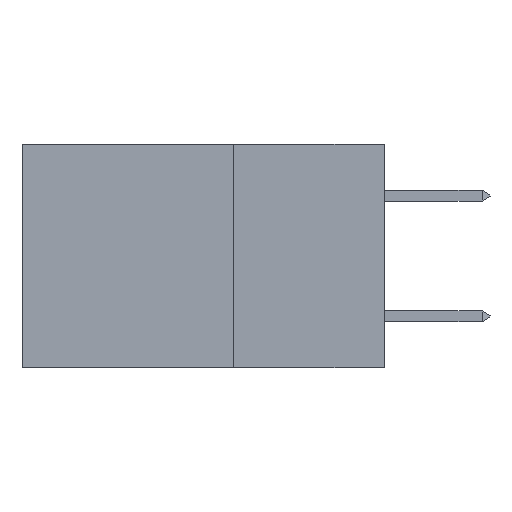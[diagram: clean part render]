
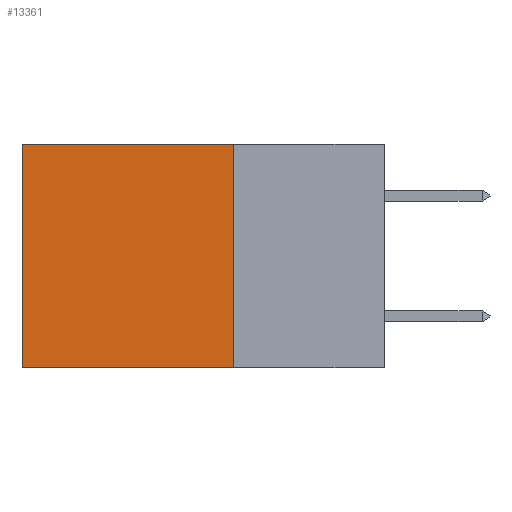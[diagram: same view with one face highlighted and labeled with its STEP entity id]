
A CAD part, left-side view. The second image highlights one B-rep face of the part: STEP entity #13361.
In plain terms, the highlighted planar face has unit normal (-1, 0, 0).
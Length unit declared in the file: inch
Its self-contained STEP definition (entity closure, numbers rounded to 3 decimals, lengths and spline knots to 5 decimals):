
#562 = PLANE ( 'NONE',  #2288 ) ;
#774 = DIRECTION ( 'NONE',  ( 0., 1., 0. ) ) ;
#834 = FACE_OUTER_BOUND ( 'NONE', #16332, .T. ) ;
#994 = ORIENTED_EDGE ( 'NONE', *, *, #23480, .T. ) ;
#1142 = VECTOR ( 'NONE', #774, 39.37008 ) ;
#2156 = CARTESIAN_POINT ( 'NONE',  ( 0.2875, 0.25, -0.37 ) ) ;
#2288 = AXIS2_PLACEMENT_3D ( 'NONE', #22268, #9350, #15527 ) ;
#2604 = CARTESIAN_POINT ( 'NONE',  ( 0.2875, 0.6, -0.37 ) ) ;
#4967 = CARTESIAN_POINT ( 'NONE',  ( 0.2875, 0.25, 0. ) ) ;
#6577 = CARTESIAN_POINT ( 'NONE',  ( 0.2875, 0.6, 0. ) ) ;
#6912 = VERTEX_POINT ( 'NONE', #2604 ) ;
#6978 = EDGE_CURVE ( 'NONE', #10164, #23298, #17303, .T. ) ;
#7109 = VECTOR ( 'NONE', #21839, 39.37008 ) ;
#7197 = VERTEX_POINT ( 'NONE', #2156 ) ;
#9350 = DIRECTION ( 'NONE',  ( 1., 0., 0. ) ) ;
#10164 = VERTEX_POINT ( 'NONE', #12067 ) ;
#11498 = ORIENTED_EDGE ( 'NONE', *, *, #21972, .F. ) ;
#12067 = CARTESIAN_POINT ( 'NONE',  ( 0.2875, 0.25, 0. ) ) ;
#12426 = VECTOR ( 'NONE', #22539, 39.37008 ) ;
#13188 = ORIENTED_EDGE ( 'NONE', *, *, #6978, .T. ) ;
#13361 = ADVANCED_FACE ( 'NONE', ( #834 ), #562, .F. ) ;
#13532 = CARTESIAN_POINT ( 'NONE',  ( 0.2875, 0.6, 0. ) ) ;
#13834 = CARTESIAN_POINT ( 'NONE',  ( 0.2875, 0.25, -0.37 ) ) ;
#14234 = VECTOR ( 'NONE', #22208, 39.37008 ) ;
#15527 = DIRECTION ( 'NONE',  ( 0., 0., -1. ) ) ;
#16153 = ORIENTED_EDGE ( 'NONE', *, *, #22851, .F. ) ;
#16332 = EDGE_LOOP ( 'NONE', ( #994, #11498, #16153, #13188 ) ) ;
#16549 = CARTESIAN_POINT ( 'NONE',  ( 0.2875, 0.25, 0. ) ) ;
#17303 = LINE ( 'NONE', #4967, #1142 ) ;
#17473 = LINE ( 'NONE', #13532, #7109 ) ;
#20903 = LINE ( 'NONE', #16549, #14234 ) ;
#21839 = DIRECTION ( 'NONE',  ( 0., 0., -1. ) ) ;
#21972 = EDGE_CURVE ( 'NONE', #7197, #6912, #24633, .T. ) ;
#22208 = DIRECTION ( 'NONE',  ( 0., 0., -1. ) ) ;
#22268 = CARTESIAN_POINT ( 'NONE',  ( 0.2875, 0.25, 0. ) ) ;
#22539 = DIRECTION ( 'NONE',  ( 0., 1., 0. ) ) ;
#22851 = EDGE_CURVE ( 'NONE', #10164, #7197, #20903, .T. ) ;
#23298 = VERTEX_POINT ( 'NONE', #6577 ) ;
#23480 = EDGE_CURVE ( 'NONE', #23298, #6912, #17473, .T. ) ;
#24633 = LINE ( 'NONE', #13834, #12426 ) ;
